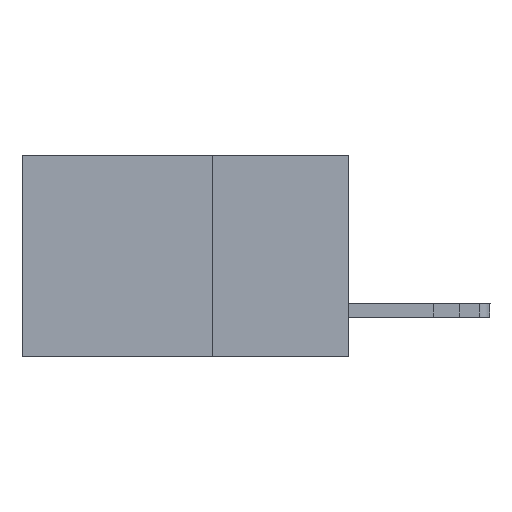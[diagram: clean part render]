
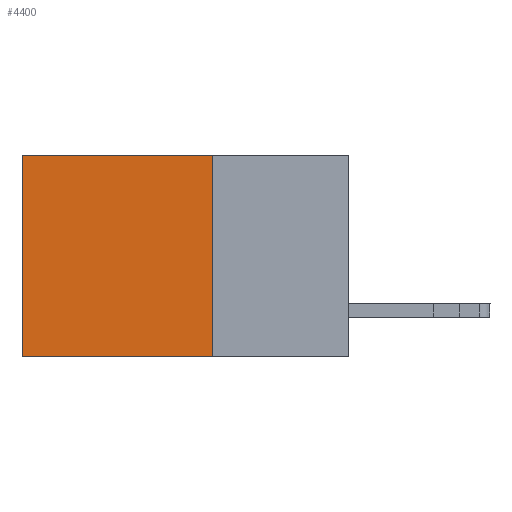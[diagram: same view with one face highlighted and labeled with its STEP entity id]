
A CAD part, left-side view. The second image highlights one B-rep face of the part: STEP entity #4400.
In plain terms, the highlighted planar face has unit normal (-1, 0, 0).
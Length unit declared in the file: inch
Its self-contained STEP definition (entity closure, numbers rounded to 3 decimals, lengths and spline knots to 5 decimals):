
#782 = VECTOR ( 'NONE', #9992, 39.37008 ) ;
#2691 = LINE ( 'NONE', #2879, #15407 ) ;
#2692 = CARTESIAN_POINT ( 'NONE',  ( 0.2615, 0.6, -0.37 ) ) ;
#2879 = CARTESIAN_POINT ( 'NONE',  ( 0.2615, 0.25, -0.37 ) ) ;
#3069 = CARTESIAN_POINT ( 'NONE',  ( 0.2615, 0.25, 0. ) ) ;
#3185 = AXIS2_PLACEMENT_3D ( 'NONE', #10653, #10559, #10374 ) ;
#3240 = DIRECTION ( 'NONE',  ( 0., 1., 0. ) ) ;
#3288 = EDGE_CURVE ( 'NONE', #13856, #7667, #16742, .T. ) ;
#3418 = ORIENTED_EDGE ( 'NONE', *, *, #17282, .F. ) ;
#4058 = CARTESIAN_POINT ( 'NONE',  ( 0.2615, 0.6, -0.37 ) ) ;
#4266 = CARTESIAN_POINT ( 'NONE',  ( 0.2615, 0.25, -0.37 ) ) ;
#4400 = ADVANCED_FACE ( 'NONE', ( #18529 ), #10807, .F. ) ;
#4641 = VERTEX_POINT ( 'NONE', #5775 ) ;
#4744 = ORIENTED_EDGE ( 'NONE', *, *, #5684, .F. ) ;
#5684 = EDGE_CURVE ( 'NONE', #4641, #7667, #15330, .T. ) ;
#5712 = ORIENTED_EDGE ( 'NONE', *, *, #7487, .T. ) ;
#5775 = CARTESIAN_POINT ( 'NONE',  ( 0.2615, 0.25, -0.37 ) ) ;
#7487 = EDGE_CURVE ( 'NONE', #9362, #13856, #9585, .T. ) ;
#7667 = VERTEX_POINT ( 'NONE', #4058 ) ;
#9362 = VERTEX_POINT ( 'NONE', #3069 ) ;
#9479 = DIRECTION ( 'NONE',  ( 0., 0., -1. ) ) ;
#9579 = CARTESIAN_POINT ( 'NONE',  ( 0.2615, 0.6, 0. ) ) ;
#9585 = LINE ( 'NONE', #10109, #782 ) ;
#9992 = DIRECTION ( 'NONE',  ( 0., 1., 0. ) ) ;
#10109 = CARTESIAN_POINT ( 'NONE',  ( 0.2615, 0.25, 0. ) ) ;
#10374 = DIRECTION ( 'NONE',  ( 0., 0., -1. ) ) ;
#10426 = VECTOR ( 'NONE', #3240, 39.37008 ) ;
#10559 = DIRECTION ( 'NONE',  ( 1., 0., 0. ) ) ;
#10653 = CARTESIAN_POINT ( 'NONE',  ( 0.2615, 0.25, -0.37 ) ) ;
#10807 = PLANE ( 'NONE',  #3185 ) ;
#13856 = VERTEX_POINT ( 'NONE', #9579 ) ;
#15330 = LINE ( 'NONE', #4266, #10426 ) ;
#15407 = VECTOR ( 'NONE', #9479, 39.37008 ) ;
#16742 = LINE ( 'NONE', #2692, #20543 ) ;
#17282 = EDGE_CURVE ( 'NONE', #9362, #4641, #2691, .T. ) ;
#18529 = FACE_OUTER_BOUND ( 'NONE', #21007, .T. ) ;
#19214 = DIRECTION ( 'NONE',  ( 0., 0., -1. ) ) ;
#20543 = VECTOR ( 'NONE', #19214, 39.37008 ) ;
#21007 = EDGE_LOOP ( 'NONE', ( #21054, #4744, #3418, #5712 ) ) ;
#21054 = ORIENTED_EDGE ( 'NONE', *, *, #3288, .T. ) ;
